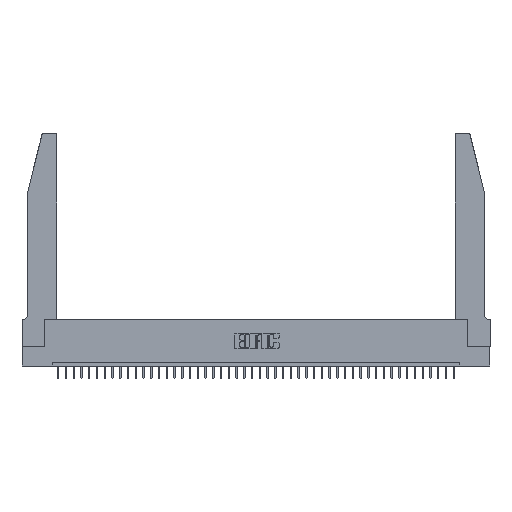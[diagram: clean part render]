
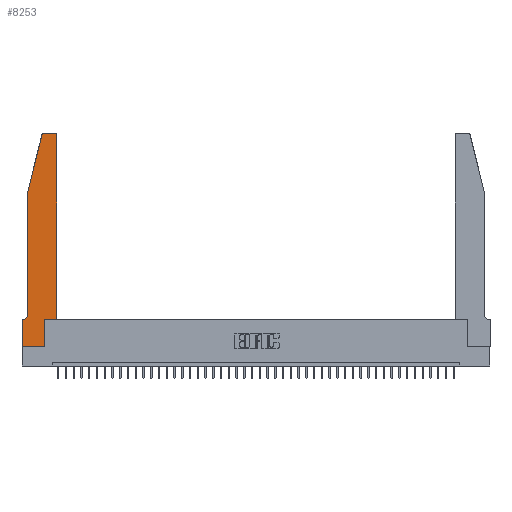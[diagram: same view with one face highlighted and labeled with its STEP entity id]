
A CAD part, top view. The second image highlights one B-rep face of the part: STEP entity #8253.
In plain terms, the highlighted planar face has unit normal (0, 0, 1).
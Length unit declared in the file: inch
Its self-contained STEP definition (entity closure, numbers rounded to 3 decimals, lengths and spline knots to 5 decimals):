
#972 = DIRECTION ( 'NONE',  ( 1., 0., 0. ) ) ;
#1074 = VECTOR ( 'NONE', #22258, 39.37008 ) ;
#1535 = FACE_OUTER_BOUND ( 'NONE', #34577, .T. ) ;
#1775 = VERTEX_POINT ( 'NONE', #13784 ) ;
#1801 = DIRECTION ( 'NONE',  ( -0.239, -0.971, 0. ) ) ;
#1855 = ORIENTED_EDGE ( 'NONE', *, *, #23002, .T. ) ;
#2401 = CARTESIAN_POINT ( 'NONE',  ( 0.0755, 0.42, 0.37 ) ) ;
#2769 = EDGE_CURVE ( 'NONE', #24406, #17012, #16422, .T. ) ;
#3048 = VERTEX_POINT ( 'NONE', #12387 ) ;
#4160 = VERTEX_POINT ( 'NONE', #9751 ) ;
#4740 = ORIENTED_EDGE ( 'NONE', *, *, #2769, .T. ) ;
#6124 = CARTESIAN_POINT ( 'NONE',  ( 0.284, 2.75, 0.37 ) ) ;
#6663 = CARTESIAN_POINT ( 'NONE',  ( 0.0055, 0.35, 0.37 ) ) ;
#7007 = DIRECTION ( 'NONE',  ( 0., 0., 1. ) ) ;
#7256 = DIRECTION ( 'NONE',  ( 0., -1., 0. ) ) ;
#7461 = AXIS2_PLACEMENT_3D ( 'NONE', #39547, #11159, #37362 ) ;
#7828 = EDGE_CURVE ( 'NONE', #17012, #3048, #16390, .T. ) ;
#8253 = ADVANCED_FACE ( 'NONE', ( #1535 ), #30179, .T. ) ;
#8631 = VERTEX_POINT ( 'NONE', #41306 ) ;
#8779 = ORIENTED_EDGE ( 'NONE', *, *, #17700, .T. ) ;
#9002 = ORIENTED_EDGE ( 'NONE', *, *, #19166, .T. ) ;
#9336 = EDGE_CURVE ( 'NONE', #30413, #8631, #25640, .T. ) ;
#9751 = CARTESIAN_POINT ( 'NONE',  ( 0.4505, 0.35, 0.37 ) ) ;
#10399 = CIRCLE ( 'NONE', #34737, 0.07 ) ;
#10446 = DIRECTION ( 'NONE',  ( -1., 0., 0. ) ) ;
#10638 = CARTESIAN_POINT ( 'NONE',  ( 0.2865, 0., 0.37 ) ) ;
#11151 = LINE ( 'NONE', #20317, #23987 ) ;
#11159 = DIRECTION ( 'NONE',  ( 0., 0., 1. ) ) ;
#11500 = CARTESIAN_POINT ( 'NONE',  ( 0.0755, 0.35, 0.37 ) ) ;
#12387 = CARTESIAN_POINT ( 'NONE',  ( 0.2865, 0.35, 0.37 ) ) ;
#13429 = LINE ( 'NONE', #14826, #39248 ) ;
#13784 = CARTESIAN_POINT ( 'NONE',  ( 0.4205, 2.75, 0.37 ) ) ;
#14242 = DIRECTION ( 'NONE',  ( 1., 0., 0. ) ) ;
#14715 = VECTOR ( 'NONE', #14242, 39.37008 ) ;
#14826 = CARTESIAN_POINT ( 'NONE',  ( 0.0755, 2., 0.37 ) ) ;
#15893 = CIRCLE ( 'NONE', #31093, 0.03 ) ;
#16207 = VERTEX_POINT ( 'NONE', #29105 ) ;
#16390 = LINE ( 'NONE', #41704, #42226 ) ;
#16422 = LINE ( 'NONE', #41529, #1074 ) ;
#16630 = VERTEX_POINT ( 'NONE', #38139 ) ;
#16847 = ORIENTED_EDGE ( 'NONE', *, *, #33175, .T. ) ;
#16875 = DIRECTION ( 'NONE',  ( 0., 0., 1. ) ) ;
#16929 = ORIENTED_EDGE ( 'NONE', *, *, #37748, .T. ) ;
#17012 = VERTEX_POINT ( 'NONE', #10638 ) ;
#17172 = CARTESIAN_POINT ( 'NONE',  ( 0.284, 2.72, 0.37 ) ) ;
#17700 = EDGE_CURVE ( 'NONE', #1775, #22806, #42031, .T. ) ;
#18635 = VERTEX_POINT ( 'NONE', #42333 ) ;
#18659 = DIRECTION ( 'NONE',  ( 0., 0., -1. ) ) ;
#19037 = VECTOR ( 'NONE', #24549, 39.37008 ) ;
#19166 = EDGE_CURVE ( 'NONE', #27032, #30413, #10399, .T. ) ;
#20317 = CARTESIAN_POINT ( 'NONE',  ( 0.0755, 2., 0.37 ) ) ;
#20762 = LINE ( 'NONE', #32384, #37283 ) ;
#21294 = EDGE_CURVE ( 'NONE', #16207, #1775, #15893, .T. ) ;
#21346 = EDGE_CURVE ( 'NONE', #22806, #18635, #34473, .T. ) ;
#21396 = ORIENTED_EDGE ( 'NONE', *, *, #7828, .T. ) ;
#21843 = ORIENTED_EDGE ( 'NONE', *, *, #23094, .T. ) ;
#22258 = DIRECTION ( 'NONE',  ( 1., 0., 0. ) ) ;
#22806 = VERTEX_POINT ( 'NONE', #6124 ) ;
#22953 = LINE ( 'NONE', #30987, #14715 ) ;
#23002 = EDGE_CURVE ( 'NONE', #16630, #27032, #11151, .T. ) ;
#23094 = EDGE_CURVE ( 'NONE', #3048, #4160, #22953, .T. ) ;
#23812 = CARTESIAN_POINT ( 'NONE',  ( 0.2605, 2.75, 0.37 ) ) ;
#23987 = VECTOR ( 'NONE', #7256, 39.37008 ) ;
#24173 = DIRECTION ( 'NONE',  ( -1., 0., 0. ) ) ;
#24406 = VERTEX_POINT ( 'NONE', #25970 ) ;
#24549 = DIRECTION ( 'NONE',  ( 0., 1., 0. ) ) ;
#25640 = LINE ( 'NONE', #11500, #28248 ) ;
#25970 = CARTESIAN_POINT ( 'NONE',  ( 0., 0., 0.37 ) ) ;
#26368 = ORIENTED_EDGE ( 'NONE', *, *, #31498, .T. ) ;
#26786 = LINE ( 'NONE', #41555, #19037 ) ;
#27032 = VERTEX_POINT ( 'NONE', #2401 ) ;
#28248 = VECTOR ( 'NONE', #24173, 39.37008 ) ;
#29105 = CARTESIAN_POINT ( 'NONE',  ( 0.4505, 2.72, 0.37 ) ) ;
#30179 = PLANE ( 'NONE',  #7461 ) ;
#30413 = VERTEX_POINT ( 'NONE', #6663 ) ;
#30987 = CARTESIAN_POINT ( 'NONE',  ( 0.4505, 0.35, 0.37 ) ) ;
#31093 = AXIS2_PLACEMENT_3D ( 'NONE', #36917, #7007, #972 ) ;
#31498 = EDGE_CURVE ( 'NONE', #8631, #24406, #20762, .T. ) ;
#32384 = CARTESIAN_POINT ( 'NONE',  ( 0., 0., 0.37 ) ) ;
#33175 = EDGE_CURVE ( 'NONE', #4160, #16207, #26786, .T. ) ;
#33256 = ORIENTED_EDGE ( 'NONE', *, *, #21294, .T. ) ;
#34473 = CIRCLE ( 'NONE', #40190, 0.03 ) ;
#34577 = EDGE_LOOP ( 'NONE', ( #8779, #35022, #16929, #1855, #9002, #38148, #26368, #4740, #21396, #21843, #16847, #33256 ) ) ;
#34737 = AXIS2_PLACEMENT_3D ( 'NONE', #35341, #18659, #42006 ) ;
#35022 = ORIENTED_EDGE ( 'NONE', *, *, #21346, .T. ) ;
#35341 = CARTESIAN_POINT ( 'NONE',  ( 0.0055, 0.42, 0.37 ) ) ;
#36917 = CARTESIAN_POINT ( 'NONE',  ( 0.4205, 2.72, 0.37 ) ) ;
#36967 = VECTOR ( 'NONE', #10446, 39.37008 ) ;
#37283 = VECTOR ( 'NONE', #42140, 39.37008 ) ;
#37362 = DIRECTION ( 'NONE',  ( 1., 0., 0. ) ) ;
#37748 = EDGE_CURVE ( 'NONE', #18635, #16630, #13429, .T. ) ;
#38139 = CARTESIAN_POINT ( 'NONE',  ( 0.0755, 2., 0.37 ) ) ;
#38148 = ORIENTED_EDGE ( 'NONE', *, *, #9336, .T. ) ;
#39101 = DIRECTION ( 'NONE',  ( 0., 1., 0. ) ) ;
#39248 = VECTOR ( 'NONE', #1801, 39.37008 ) ;
#39547 = CARTESIAN_POINT ( 'NONE',  ( 0., 0.35, 0.37 ) ) ;
#39982 = DIRECTION ( 'NONE',  ( 1., 0., 0. ) ) ;
#40190 = AXIS2_PLACEMENT_3D ( 'NONE', #17172, #16875, #39982 ) ;
#41306 = CARTESIAN_POINT ( 'NONE',  ( 0., 0.35, 0.37 ) ) ;
#41529 = CARTESIAN_POINT ( 'NONE',  ( 0., 0., 0.37 ) ) ;
#41555 = CARTESIAN_POINT ( 'NONE',  ( 0.4505, 0.35, 0.37 ) ) ;
#41704 = CARTESIAN_POINT ( 'NONE',  ( 0.2865, 0.35, 0.37 ) ) ;
#42006 = DIRECTION ( 'NONE',  ( -1., 0., 0. ) ) ;
#42031 = LINE ( 'NONE', #23812, #36967 ) ;
#42140 = DIRECTION ( 'NONE',  ( 0., -1., 0. ) ) ;
#42226 = VECTOR ( 'NONE', #39101, 39.37008 ) ;
#42333 = CARTESIAN_POINT ( 'NONE',  ( 0.25487, 2.72718, 0.37 ) ) ;
